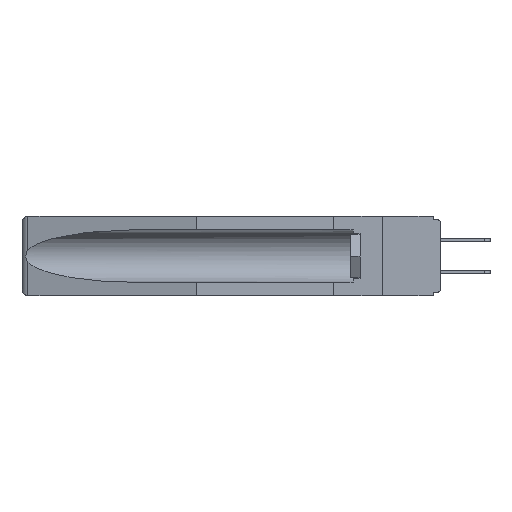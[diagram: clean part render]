
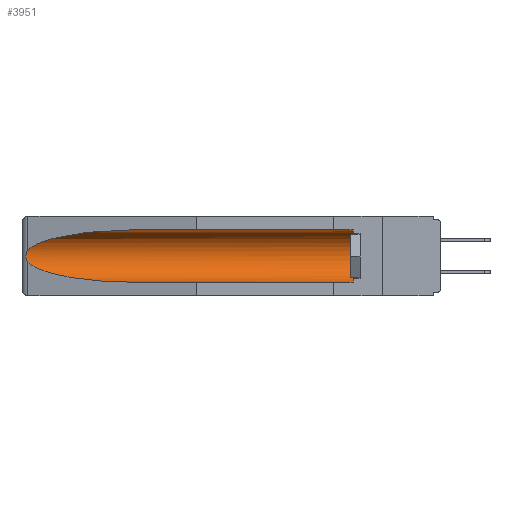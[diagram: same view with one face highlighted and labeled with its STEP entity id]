
A CAD part, left-side view. The second image highlights one B-rep face of the part: STEP entity #3951.
In plain terms, the highlighted cylindrical face has radius 2.857 mm (diameter 5.715 mm), a partial arc.
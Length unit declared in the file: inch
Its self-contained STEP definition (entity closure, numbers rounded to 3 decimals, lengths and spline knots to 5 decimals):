
#548 = CYLINDRICAL_SURFACE ( 'NONE', #11749, 0.1125 ) ;
#770 = CARTESIAN_POINT ( 'NONE',  ( 0.21114, 1.30732, -0.059 ) ) ;
#1062 = CARTESIAN_POINT ( 'NONE',  ( 0.26537, 1.52718, -0.14972 ) ) ;
#1881 = B_SPLINE_CURVE_WITH_KNOTS ( 'NONE', 3,
 ( #14703, #16742, #20909, #16651, #4436, #14621, #12293, #21937, #24826, #6669 ),
 .UNSPECIFIED., .F., .F.,
 ( 4, 2, 2, 2, 4 ),
 ( 0., 0.00029, 0.00058, 0.00087, 0.00117 ),
 .UNSPECIFIED. ) ;
#2073 = EDGE_CURVE ( 'NONE', #20430, #16189, #1881, .T. ) ;
#2769 = ORIENTED_EDGE ( 'NONE', *, *, #26602, .T. ) ;
#2938 = EDGE_CURVE ( 'NONE', #3060, #13568, #3150, .T. ) ;
#3060 = VERTEX_POINT ( 'NONE', #15085 ) ;
#3150 = CIRCLE ( 'NONE', #8774, 0.1125 ) ;
#3249 = EDGE_CURVE ( 'NONE', #3060, #3479, #26365, .T. ) ;
#3479 = VERTEX_POINT ( 'NONE', #25000 ) ;
#3744 = DIRECTION ( 'NONE',  ( 0., -1., 0. ) ) ;
#3951 = ADVANCED_FACE ( 'NONE', ( #8272 ), #548, .F. ) ;
#3958 = VECTOR ( 'NONE', #6708, 39.37008 ) ;
#4436 = CARTESIAN_POINT ( 'NONE',  ( 0.2675, 1.53308, -0.16763 ) ) ;
#4837 = CARTESIAN_POINT ( 'NONE',  ( 0.155, 1.07973, -0.059 ) ) ;
#5001 = ORIENTED_EDGE ( 'NONE', *, *, #2938, .T. ) ;
#5466 =( BOUNDED_CURVE ( )  B_SPLINE_CURVE ( 3, ( #4837, #770, #15020, #19436 ),
 .UNSPECIFIED., .F., .F. ) 
 B_SPLINE_CURVE_WITH_KNOTS ( ( 4, 4 ),
 ( 4.71239, 6.08839 ),
 .UNSPECIFIED. ) 
 CURVE ( )  GEOMETRIC_REPRESENTATION_ITEM ( )  RATIONAL_B_SPLINE_CURVE ( ( 1., 0.848, 0.848, 1. ) ) 
 REPRESENTATION_ITEM ( '' )  );
#6352 = EDGE_CURVE ( 'NONE', #13568, #9049, #22972, .T. ) ;
#6669 = CARTESIAN_POINT ( 'NONE',  ( 0.26537, 1.52718, -0.19328 ) ) ;
#6708 = DIRECTION ( 'NONE',  ( 0., 1., 0. ) ) ;
#7080 = CARTESIAN_POINT ( 'NONE',  ( 0.155, 0.126, -0.059 ) ) ;
#7246 = CARTESIAN_POINT ( 'NONE',  ( 0.26537, 1.52718, -0.19328 ) ) ;
#7788 =( BOUNDED_CURVE ( )  B_SPLINE_CURVE ( 3, ( #21349, #15149, #21447, #12817 ),
 .UNSPECIFIED., .F., .F. ) 
 B_SPLINE_CURVE_WITH_KNOTS ( ( 4, 4 ),
 ( 0.1948, 1.5708 ),
 .UNSPECIFIED. ) 
 CURVE ( )  GEOMETRIC_REPRESENTATION_ITEM ( )  RATIONAL_B_SPLINE_CURVE ( ( 1., 0.848, 0.848, 1. ) ) 
 REPRESENTATION_ITEM ( '' )  );
#8272 = FACE_OUTER_BOUND ( 'NONE', #21158, .T. ) ;
#8379 = ORIENTED_EDGE ( 'NONE', *, *, #2073, .T. ) ;
#8774 = AXIS2_PLACEMENT_3D ( 'NONE', #16138, #3744, #26101 ) ;
#9049 = VERTEX_POINT ( 'NONE', #13234 ) ;
#9725 = CARTESIAN_POINT ( 'NONE',  ( 0.155, -0.30754, -0.1715 ) ) ;
#9819 = DIRECTION ( 'NONE',  ( 0., 1., 0. ) ) ;
#11749 = AXIS2_PLACEMENT_3D ( 'NONE', #9725, #9819, #13888 ) ;
#12293 = CARTESIAN_POINT ( 'NONE',  ( 0.2673, 1.53269, -0.17917 ) ) ;
#12301 = ORIENTED_EDGE ( 'NONE', *, *, #6352, .T. ) ;
#12528 = VECTOR ( 'NONE', #21913, 39.37008 ) ;
#12817 = CARTESIAN_POINT ( 'NONE',  ( 0.155, 1.07973, -0.284 ) ) ;
#12855 = CARTESIAN_POINT ( 'NONE',  ( 0.155, -0.30754, -0.059 ) ) ;
#13234 = CARTESIAN_POINT ( 'NONE',  ( 0.155, 1.07973, -0.059 ) ) ;
#13568 = VERTEX_POINT ( 'NONE', #7080 ) ;
#13888 = DIRECTION ( 'NONE',  ( 0., 0., 1. ) ) ;
#14059 = EDGE_CURVE ( 'NONE', #16189, #3479, #7788, .T. ) ;
#14621 = CARTESIAN_POINT ( 'NONE',  ( 0.2675, 1.53308, -0.17534 ) ) ;
#14703 = CARTESIAN_POINT ( 'NONE',  ( 0.26537, 1.52718, -0.14972 ) ) ;
#15020 = CARTESIAN_POINT ( 'NONE',  ( 0.25451, 1.48313, -0.09465 ) ) ;
#15085 = CARTESIAN_POINT ( 'NONE',  ( 0.155, 0.126, -0.284 ) ) ;
#15149 = CARTESIAN_POINT ( 'NONE',  ( 0.25451, 1.48313, -0.24835 ) ) ;
#15392 = ORIENTED_EDGE ( 'NONE', *, *, #14059, .T. ) ;
#15490 = ORIENTED_EDGE ( 'NONE', *, *, #3249, .F. ) ;
#16138 = CARTESIAN_POINT ( 'NONE',  ( 0.155, 0.126, -0.1715 ) ) ;
#16189 = VERTEX_POINT ( 'NONE', #7246 ) ;
#16651 = CARTESIAN_POINT ( 'NONE',  ( 0.2673, 1.5327, -0.16383 ) ) ;
#16742 = CARTESIAN_POINT ( 'NONE',  ( 0.26597, 1.52961, -0.15275 ) ) ;
#19436 = CARTESIAN_POINT ( 'NONE',  ( 0.26537, 1.52718, -0.14972 ) ) ;
#20430 = VERTEX_POINT ( 'NONE', #1062 ) ;
#20909 = CARTESIAN_POINT ( 'NONE',  ( 0.26654, 1.53092, -0.15636 ) ) ;
#21158 = EDGE_LOOP ( 'NONE', ( #2769, #8379, #15392, #15490, #5001, #12301 ) ) ;
#21349 = CARTESIAN_POINT ( 'NONE',  ( 0.26537, 1.52718, -0.19328 ) ) ;
#21447 = CARTESIAN_POINT ( 'NONE',  ( 0.21114, 1.30732, -0.284 ) ) ;
#21913 = DIRECTION ( 'NONE',  ( 0., 1., 0. ) ) ;
#21937 = CARTESIAN_POINT ( 'NONE',  ( 0.26655, 1.53094, -0.18657 ) ) ;
#22972 = LINE ( 'NONE', #12855, #3958 ) ;
#24826 = CARTESIAN_POINT ( 'NONE',  ( 0.26597, 1.5296, -0.19026 ) ) ;
#25000 = CARTESIAN_POINT ( 'NONE',  ( 0.155, 1.07973, -0.284 ) ) ;
#25967 = CARTESIAN_POINT ( 'NONE',  ( 0.155, -0.30754, -0.284 ) ) ;
#26101 = DIRECTION ( 'NONE',  ( 0., 0., 1. ) ) ;
#26365 = LINE ( 'NONE', #25967, #12528 ) ;
#26602 = EDGE_CURVE ( 'NONE', #9049, #20430, #5466, .T. ) ;
